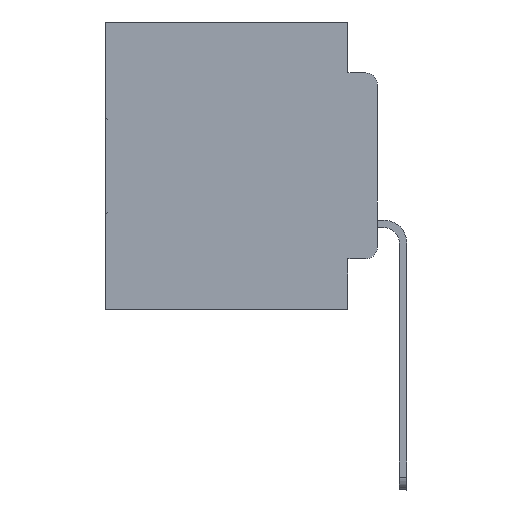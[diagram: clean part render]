
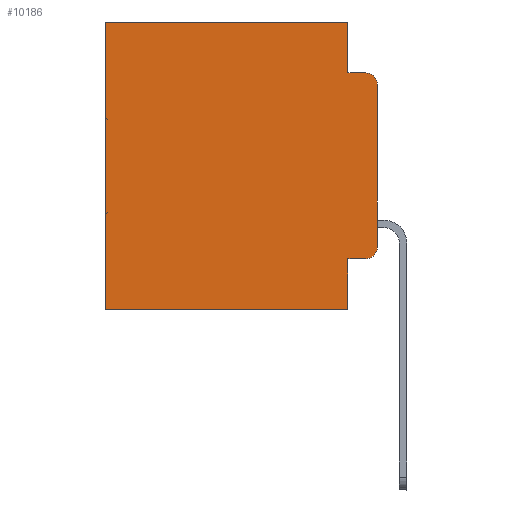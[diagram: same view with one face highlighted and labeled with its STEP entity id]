
A CAD part, left-side view. The second image highlights one B-rep face of the part: STEP entity #10186.
In plain terms, the highlighted planar face has unit normal (-1, 0, 0).
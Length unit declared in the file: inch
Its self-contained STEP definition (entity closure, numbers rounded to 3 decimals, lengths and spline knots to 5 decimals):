
#763 = CARTESIAN_POINT ( 'NONE',  ( 0.298, 0.02, -0.1085 ) ) ;
#831 = CARTESIAN_POINT ( 'NONE',  ( 0.298, 0., 0. ) ) ;
#1950 = DIRECTION ( 'NONE',  ( 0., 0., -1. ) ) ;
#2526 = LINE ( 'NONE', #12297, #13061 ) ;
#2629 = ORIENTED_EDGE ( 'NONE', *, *, #12845, .T. ) ;
#2921 = DIRECTION ( 'NONE',  ( 0., -1., 0. ) ) ;
#3003 = VERTEX_POINT ( 'NONE', #30457 ) ;
#3066 = AXIS2_PLACEMENT_3D ( 'NONE', #30459, #27607, #20270 ) ;
#3088 = VECTOR ( 'NONE', #26395, 39.37008 ) ;
#3439 = CARTESIAN_POINT ( 'NONE',  ( 0.298, 0., 0. ) ) ;
#3490 = VERTEX_POINT ( 'NONE', #27818 ) ;
#3801 = AXIS2_PLACEMENT_3D ( 'NONE', #15011, #4325, #1950 ) ;
#3908 = CARTESIAN_POINT ( 'NONE',  ( 0.298, 0.051, 0. ) ) ;
#4127 = CARTESIAN_POINT ( 'NONE',  ( 0.298, 0.051, -0.5 ) ) ;
#4325 = DIRECTION ( 'NONE',  ( 1., 0., 0. ) ) ;
#4446 = CARTESIAN_POINT ( 'NONE',  ( 0.298, 0.02, -0.4115 ) ) ;
#5302 = VERTEX_POINT ( 'NONE', #10300 ) ;
#5744 = CARTESIAN_POINT ( 'NONE',  ( 0.298, 0.051, 0. ) ) ;
#6486 = VECTOR ( 'NONE', #2921, 39.37008 ) ;
#6520 = LINE ( 'NONE', #19488, #19547 ) ;
#7180 = VECTOR ( 'NONE', #14692, 39.37008 ) ;
#8730 = VECTOR ( 'NONE', #24856, 39.37008 ) ;
#9164 = EDGE_CURVE ( 'NONE', #3003, #29018, #20328, .T. ) ;
#9373 = ORIENTED_EDGE ( 'NONE', *, *, #9708, .F. ) ;
#9708 = EDGE_CURVE ( 'NONE', #16864, #24443, #31202, .T. ) ;
#10019 = LINE ( 'NONE', #831, #7180 ) ;
#10035 = CARTESIAN_POINT ( 'NONE',  ( 0.298, 0.02, -0.0885 ) ) ;
#10186 = ADVANCED_FACE ( 'NONE', ( #32836 ), #14678, .F. ) ;
#10300 = CARTESIAN_POINT ( 'NONE',  ( 0.298, 0.473, 0. ) ) ;
#10962 = AXIS2_PLACEMENT_3D ( 'NONE', #763, #21364, #26773 ) ;
#11683 = EDGE_CURVE ( 'NONE', #16815, #5302, #28677, .T. ) ;
#12297 = CARTESIAN_POINT ( 'NONE',  ( 0.298, 0., -0.5 ) ) ;
#12642 = CARTESIAN_POINT ( 'NONE',  ( 0.298, 0.051, 0. ) ) ;
#12845 = EDGE_CURVE ( 'NONE', #5302, #28993, #25368, .T. ) ;
#13061 = VECTOR ( 'NONE', #33068, 39.37008 ) ;
#13109 = ORIENTED_EDGE ( 'NONE', *, *, #22126, .F. ) ;
#14678 = PLANE ( 'NONE',  #3801 ) ;
#14692 = DIRECTION ( 'NONE',  ( 0., 0., -1. ) ) ;
#15011 = CARTESIAN_POINT ( 'NONE',  ( 0.298, 0., 0. ) ) ;
#15152 = DIRECTION ( 'NONE',  ( 0., 0., -1. ) ) ;
#15602 = CARTESIAN_POINT ( 'NONE',  ( 0.298, 0.473, -0.5 ) ) ;
#15669 = CARTESIAN_POINT ( 'NONE',  ( 0.298, 0.051, -0.0885 ) ) ;
#15754 = EDGE_CURVE ( 'NONE', #16864, #17790, #6520, .T. ) ;
#15959 = EDGE_CURVE ( 'NONE', #17790, #19266, #24395, .T. ) ;
#16604 = ORIENTED_EDGE ( 'NONE', *, *, #15754, .T. ) ;
#16815 = VERTEX_POINT ( 'NONE', #5744 ) ;
#16864 = VERTEX_POINT ( 'NONE', #29484 ) ;
#17031 = EDGE_CURVE ( 'NONE', #16815, #3003, #26193, .T. ) ;
#17257 = CARTESIAN_POINT ( 'NONE',  ( 0.298, 0., -0.3915 ) ) ;
#17790 = VERTEX_POINT ( 'NONE', #4446 ) ;
#18251 = EDGE_CURVE ( 'NONE', #24443, #28993, #2526, .T. ) ;
#19118 = EDGE_CURVE ( 'NONE', #3490, #29018, #25226, .T. ) ;
#19266 = VERTEX_POINT ( 'NONE', #17257 ) ;
#19488 = CARTESIAN_POINT ( 'NONE',  ( 0.298, 0.051, -0.4115 ) ) ;
#19547 = VECTOR ( 'NONE', #21969, 39.37008 ) ;
#20260 = VECTOR ( 'NONE', #23135, 39.37008 ) ;
#20270 = DIRECTION ( 'NONE',  ( 0., 0., -1. ) ) ;
#20328 = LINE ( 'NONE', #15669, #6486 ) ;
#20423 = ORIENTED_EDGE ( 'NONE', *, *, #11683, .T. ) ;
#21364 = DIRECTION ( 'NONE',  ( -1., 0., 0. ) ) ;
#21805 = ORIENTED_EDGE ( 'NONE', *, *, #19118, .T. ) ;
#21969 = DIRECTION ( 'NONE',  ( 0., -1., 0. ) ) ;
#22014 = EDGE_LOOP ( 'NONE', ( #13109, #21805, #33381, #26236, #20423, #2629, #32243, #9373, #16604, #23809 ) ) ;
#22126 = EDGE_CURVE ( 'NONE', #3490, #19266, #10019, .T. ) ;
#23135 = DIRECTION ( 'NONE',  ( 0., 0., -1. ) ) ;
#23809 = ORIENTED_EDGE ( 'NONE', *, *, #15959, .T. ) ;
#24395 = CIRCLE ( 'NONE', #3066, 0.02 ) ;
#24443 = VERTEX_POINT ( 'NONE', #4127 ) ;
#24856 = DIRECTION ( 'NONE',  ( 0., 0., -1. ) ) ;
#25157 = CARTESIAN_POINT ( 'NONE',  ( 0.298, 0.473, 0. ) ) ;
#25226 = CIRCLE ( 'NONE', #10962, 0.02 ) ;
#25368 = LINE ( 'NONE', #25157, #28621 ) ;
#26193 = LINE ( 'NONE', #3908, #8730 ) ;
#26236 = ORIENTED_EDGE ( 'NONE', *, *, #17031, .F. ) ;
#26395 = DIRECTION ( 'NONE',  ( 0., 1., 0. ) ) ;
#26773 = DIRECTION ( 'NONE',  ( 0., 0., -1. ) ) ;
#27607 = DIRECTION ( 'NONE',  ( -1., 0., 0. ) ) ;
#27818 = CARTESIAN_POINT ( 'NONE',  ( 0.298, 0., -0.1085 ) ) ;
#28621 = VECTOR ( 'NONE', #15152, 39.37008 ) ;
#28677 = LINE ( 'NONE', #3439, #3088 ) ;
#28993 = VERTEX_POINT ( 'NONE', #15602 ) ;
#29018 = VERTEX_POINT ( 'NONE', #10035 ) ;
#29484 = CARTESIAN_POINT ( 'NONE',  ( 0.298, 0.051, -0.4115 ) ) ;
#30457 = CARTESIAN_POINT ( 'NONE',  ( 0.298, 0.051, -0.0885 ) ) ;
#30459 = CARTESIAN_POINT ( 'NONE',  ( 0.298, 0.02, -0.3915 ) ) ;
#31202 = LINE ( 'NONE', #12642, #20260 ) ;
#32243 = ORIENTED_EDGE ( 'NONE', *, *, #18251, .F. ) ;
#32836 = FACE_OUTER_BOUND ( 'NONE', #22014, .T. ) ;
#33068 = DIRECTION ( 'NONE',  ( 0., 1., 0. ) ) ;
#33381 = ORIENTED_EDGE ( 'NONE', *, *, #9164, .F. ) ;
